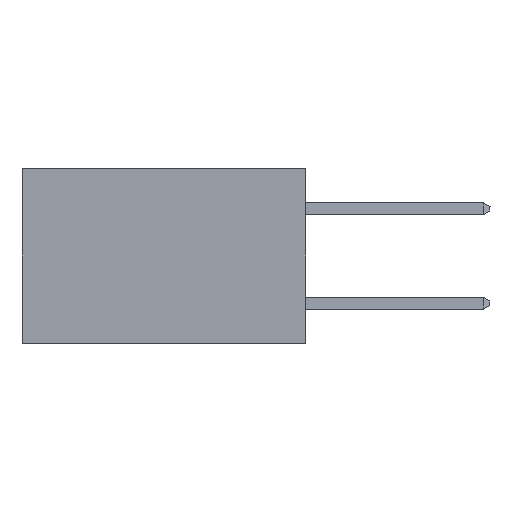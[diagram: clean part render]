
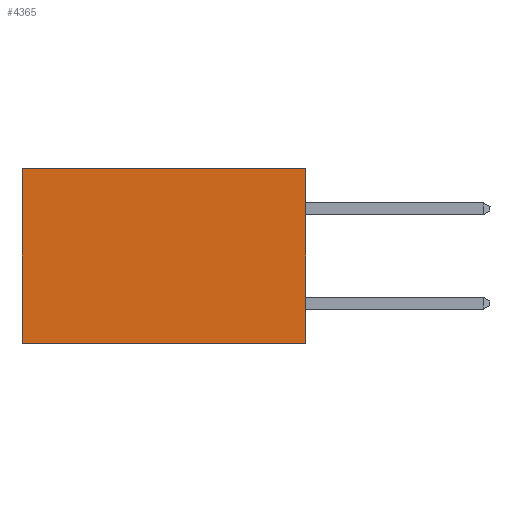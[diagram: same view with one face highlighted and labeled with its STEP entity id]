
A CAD part, left-side view. The second image highlights one B-rep face of the part: STEP entity #4365.
In plain terms, the highlighted planar face has unit normal (-1, 0, 0).
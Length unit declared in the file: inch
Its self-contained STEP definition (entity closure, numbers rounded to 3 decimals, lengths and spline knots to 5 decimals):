
#584 = DIRECTION ( 'NONE',  ( 0., 0., -1. ) ) ;
#1150 = AXIS2_PLACEMENT_3D ( 'NONE', #4154, #8763, #584 ) ;
#1167 = EDGE_CURVE ( 'NONE', #6625, #8246, #3239, .T. ) ;
#2256 = LINE ( 'NONE', #9677, #3536 ) ;
#2326 = VECTOR ( 'NONE', #10410, 39.37008 ) ;
#2396 = DIRECTION ( 'NONE',  ( 0., 1., 0. ) ) ;
#2508 = PLANE ( 'NONE',  #1150 ) ;
#2567 = DIRECTION ( 'NONE',  ( 0., 0., -1. ) ) ;
#2696 = CARTESIAN_POINT ( 'NONE',  ( 0.298, 0., -0.37 ) ) ;
#3239 = LINE ( 'NONE', #11445, #11241 ) ;
#3536 = VECTOR ( 'NONE', #2396, 39.37008 ) ;
#4154 = CARTESIAN_POINT ( 'NONE',  ( 0.298, 0., 0. ) ) ;
#4365 = ADVANCED_FACE ( 'NONE', ( #5660 ), #2508, .F. ) ;
#5047 = EDGE_CURVE ( 'NONE', #9265, #5732, #7910, .T. ) ;
#5557 = CARTESIAN_POINT ( 'NONE',  ( 0.298, 0.6, -0.37 ) ) ;
#5561 = ORIENTED_EDGE ( 'NONE', *, *, #6648, .F. ) ;
#5660 = FACE_OUTER_BOUND ( 'NONE', #6223, .T. ) ;
#5732 = VERTEX_POINT ( 'NONE', #5557 ) ;
#6223 = EDGE_LOOP ( 'NONE', ( #10329, #5561, #8277, #9067 ) ) ;
#6625 = VERTEX_POINT ( 'NONE', #9517 ) ;
#6648 = EDGE_CURVE ( 'NONE', #8246, #5732, #2256, .T. ) ;
#6739 = CARTESIAN_POINT ( 'NONE',  ( 0.298, 0.6, 0. ) ) ;
#7886 = CARTESIAN_POINT ( 'NONE',  ( 0.298, 0.6, 0. ) ) ;
#7910 = LINE ( 'NONE', #7886, #11154 ) ;
#7935 = LINE ( 'NONE', #9637, #2326 ) ;
#8246 = VERTEX_POINT ( 'NONE', #2696 ) ;
#8277 = ORIENTED_EDGE ( 'NONE', *, *, #1167, .F. ) ;
#8763 = DIRECTION ( 'NONE',  ( 1., 0., 0. ) ) ;
#9067 = ORIENTED_EDGE ( 'NONE', *, *, #10529, .T. ) ;
#9265 = VERTEX_POINT ( 'NONE', #6739 ) ;
#9517 = CARTESIAN_POINT ( 'NONE',  ( 0.298, 0., 0. ) ) ;
#9637 = CARTESIAN_POINT ( 'NONE',  ( 0.298, 0., 0. ) ) ;
#9654 = DIRECTION ( 'NONE',  ( 0., 0., -1. ) ) ;
#9677 = CARTESIAN_POINT ( 'NONE',  ( 0.298, 0., -0.37 ) ) ;
#10329 = ORIENTED_EDGE ( 'NONE', *, *, #5047, .T. ) ;
#10410 = DIRECTION ( 'NONE',  ( 0., 1., 0. ) ) ;
#10529 = EDGE_CURVE ( 'NONE', #6625, #9265, #7935, .T. ) ;
#11154 = VECTOR ( 'NONE', #9654, 39.37008 ) ;
#11241 = VECTOR ( 'NONE', #2567, 39.37008 ) ;
#11445 = CARTESIAN_POINT ( 'NONE',  ( 0.298, 0., 0. ) ) ;
